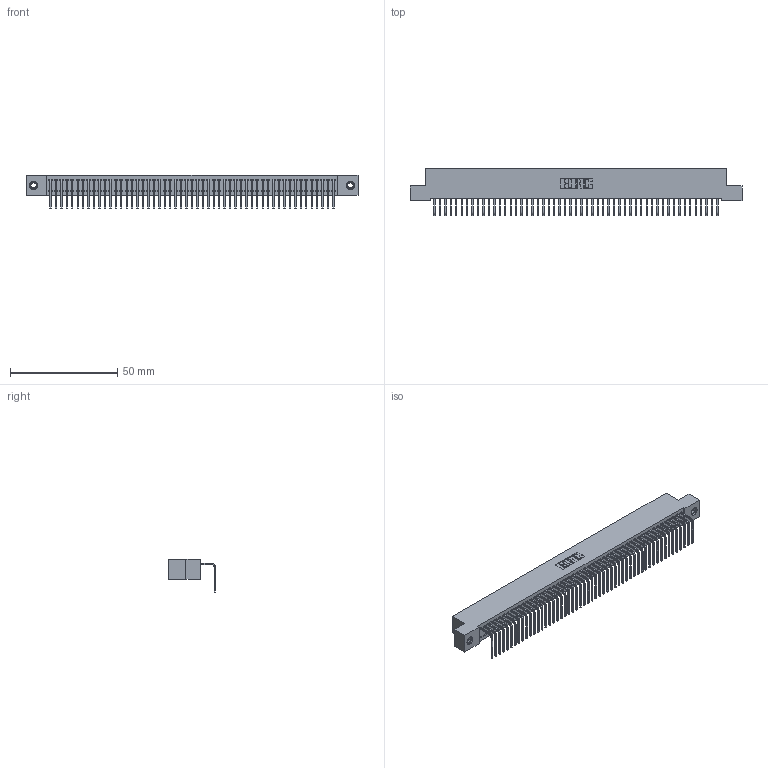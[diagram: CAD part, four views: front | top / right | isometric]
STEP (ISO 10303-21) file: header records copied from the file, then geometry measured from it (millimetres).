
FILE_DESCRIPTION (( 'STEP AP203' ), '1' );
FILE_NAME ('392-053-558-107.STEP', '2018-08-17T07:48:23', ( '' ), ( '' ), 'SwSTEP 2.0', 'SolidWorks 2016', '' );
FILE_SCHEMA (( 'CONFIG_CONTROL_DESIGN' ));
Length unit declared in the file: inch
Products named in the file (4): 342 Part_TI; 345-292-001_558 Tail - 2; 345-250-001_345-250-005-103; 392-053-558-107
Assembly tree (56 placements, depth 2):
  392-053-558-107
    342 Part_TI
    345-292-001_558 Tail - 2  x53
    345-250-001_345-250-005-103  x2
Bounding box: 154.94 x 21.91 x 15.62 mm (x, y, z)
Volume: 13789.6 mm3; surface area: 21489.8 mm2
Topology: 56 solids, 56 shells, 3350 faces, 10081 edges, 6642 vertices
Faces by surface type: plane 2430, cylinder 904, cone 12, torus 4
Entity records: 32116 total; most frequent: CARTESIAN_POINT 5520, ORIENTED_EDGE 5502, DIRECTION 4667, EDGE_CURVE 2751, LINE 2603, VECTOR 2603, VERTEX_POINT 1828, AXIS2_PLACEMENT_3D 1032
